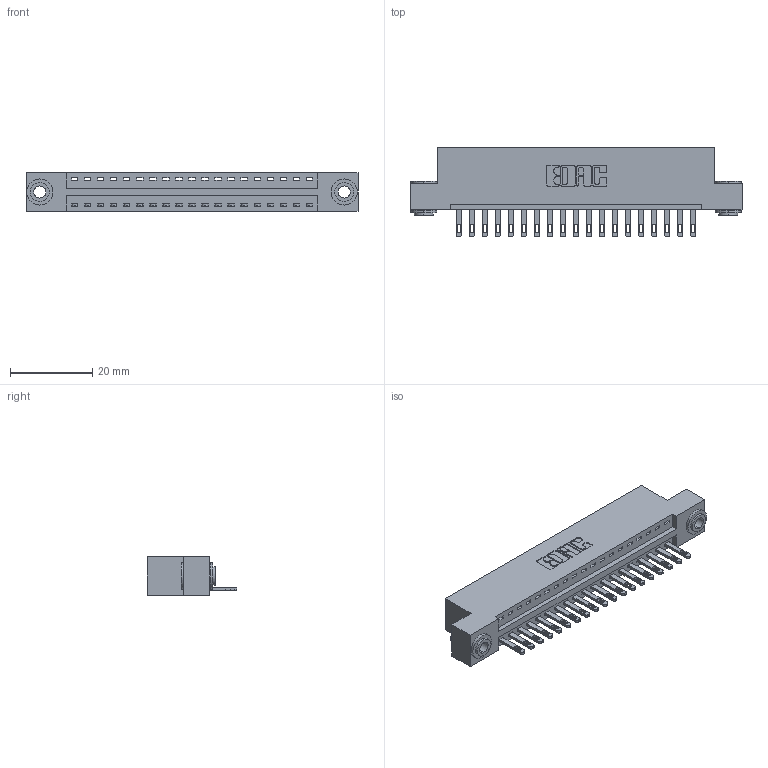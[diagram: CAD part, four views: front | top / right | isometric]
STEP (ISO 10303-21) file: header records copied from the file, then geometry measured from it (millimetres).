
FILE_DESCRIPTION (( 'STEP AP203' ), '1' );
FILE_NAME ('346-019-500-103.STEP', '2022-05-05T14:48:09', ( '' ), ( '' ), 'SwSTEP 2.0', 'SolidWorks 2020', '' );
FILE_SCHEMA (( 'CONFIG_CONTROL_DESIGN' ));
Length unit declared in the file: inch
Products named in the file (4): 346-019-500-103; 345-250-002_345-250-002-102; 346 Part_Flush Mounting Lugs - 0.156 Dia-TH; 345-292-001_345-293-100
Assembly tree (22 placements, depth 2):
  346-019-500-103
    346 Part_Flush Mounting Lugs - 0.156 Dia-TH
    345-292-001_345-293-100  x19
    345-250-002_345-250-002-102  x2
Bounding box: 80.9 x 21.84 x 9.4 mm (x, y, z)
Volume: 7598.4 mm3; surface area: 9544.6 mm2
Topology: 22 solids, 22 shells, 1200 faces, 3633 edges, 2418 vertices
Faces by surface type: plane 746, cylinder 446, cone 8
Entity records: 15884 total; most frequent: CARTESIAN_POINT 2710, ORIENTED_EDGE 2654, DIRECTION 2451, EDGE_CURVE 1327, VECTOR 1091, LINE 1091, VERTEX_POINT 882, AXIS2_PLACEMENT_3D 680
